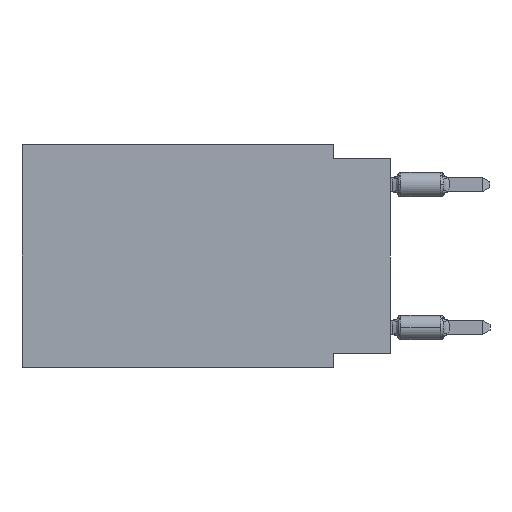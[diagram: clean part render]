
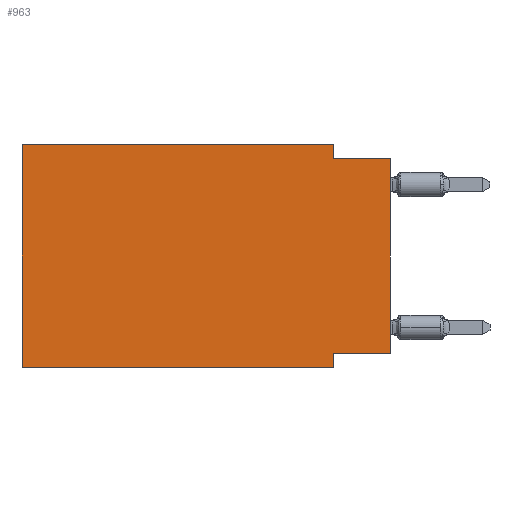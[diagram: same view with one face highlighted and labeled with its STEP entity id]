
A CAD part, left-side view. The second image highlights one B-rep face of the part: STEP entity #963.
In plain terms, the highlighted planar face has unit normal (-1, 0, 0).
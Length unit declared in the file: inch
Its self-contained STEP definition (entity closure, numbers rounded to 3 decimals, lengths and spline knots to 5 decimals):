
#391 = VECTOR ( 'NONE', #8137, 39.37008 ) ;
#597 = VERTEX_POINT ( 'NONE', #22170 ) ;
#775 = CARTESIAN_POINT ( 'NONE',  ( 0., 0.1, -0.39 ) ) ;
#792 = LINE ( 'NONE', #24409, #11663 ) ;
#963 = ADVANCED_FACE ( 'NONE', ( #3192 ), #23662, .F. ) ;
#1130 = DIRECTION ( 'NONE',  ( 0., 0., -1. ) ) ;
#1485 = EDGE_CURVE ( 'NONE', #597, #14681, #17354, .T. ) ;
#1798 = CARTESIAN_POINT ( 'NONE',  ( 0., 0., -0.025 ) ) ;
#2498 = CARTESIAN_POINT ( 'NONE',  ( 0., 0., -0.025 ) ) ;
#2582 = VECTOR ( 'NONE', #13670, 39.37008 ) ;
#2862 = LINE ( 'NONE', #9159, #14213 ) ;
#2925 = ORIENTED_EDGE ( 'NONE', *, *, #15791, .F. ) ;
#3075 = ORIENTED_EDGE ( 'NONE', *, *, #6702, .F. ) ;
#3192 = FACE_OUTER_BOUND ( 'NONE', #8140, .T. ) ;
#4168 = EDGE_CURVE ( 'NONE', #7284, #597, #2862, .T. ) ;
#5283 = LINE ( 'NONE', #15876, #2582 ) ;
#6188 = VECTOR ( 'NONE', #20323, 39.37008 ) ;
#6349 = ORIENTED_EDGE ( 'NONE', *, *, #4168, .F. ) ;
#6597 = CARTESIAN_POINT ( 'NONE',  ( 0., 0.645, -0.39 ) ) ;
#6702 = EDGE_CURVE ( 'NONE', #25868, #7284, #792, .T. ) ;
#7284 = VERTEX_POINT ( 'NONE', #14746 ) ;
#8018 = ORIENTED_EDGE ( 'NONE', *, *, #22584, .T. ) ;
#8137 = DIRECTION ( 'NONE',  ( 0., 1., 0. ) ) ;
#8140 = EDGE_LOOP ( 'NONE', ( #9874, #23512, #26373, #6349, #3075, #8018, #24072, #2925 ) ) ;
#9159 = CARTESIAN_POINT ( 'NONE',  ( 0., 0.645, 0. ) ) ;
#9247 = VERTEX_POINT ( 'NONE', #2498 ) ;
#9703 = DIRECTION ( 'NONE',  ( 0., 0., 1. ) ) ;
#9874 = ORIENTED_EDGE ( 'NONE', *, *, #14035, .T. ) ;
#10467 = CARTESIAN_POINT ( 'NONE',  ( 0., 0., -0.365 ) ) ;
#11663 = VECTOR ( 'NONE', #9703, 39.37008 ) ;
#13018 = VERTEX_POINT ( 'NONE', #22357 ) ;
#13092 = DIRECTION ( 'NONE',  ( 0., 0., -1. ) ) ;
#13108 = EDGE_CURVE ( 'NONE', #15717, #13018, #13531, .T. ) ;
#13531 = LINE ( 'NONE', #775, #24047 ) ;
#13670 = DIRECTION ( 'NONE',  ( 0., 0., 1. ) ) ;
#14035 = EDGE_CURVE ( 'NONE', #26486, #9247, #5283, .T. ) ;
#14213 = VECTOR ( 'NONE', #17275, 39.37008 ) ;
#14681 = VERTEX_POINT ( 'NONE', #20636 ) ;
#14746 = CARTESIAN_POINT ( 'NONE',  ( 0., 0.645, 0. ) ) ;
#15717 = VERTEX_POINT ( 'NONE', #18314 ) ;
#15791 = EDGE_CURVE ( 'NONE', #26486, #15717, #22843, .T. ) ;
#15876 = CARTESIAN_POINT ( 'NONE',  ( 0., 0., 0. ) ) ;
#17275 = DIRECTION ( 'NONE',  ( 0., -1., 0. ) ) ;
#17354 = LINE ( 'NONE', #25895, #23177 ) ;
#17622 = CARTESIAN_POINT ( 'NONE',  ( 0., 0.645, 0. ) ) ;
#18314 = CARTESIAN_POINT ( 'NONE',  ( 0., 0.1, -0.365 ) ) ;
#18888 = DIRECTION ( 'NONE',  ( 0., -1., 0. ) ) ;
#19033 = LINE ( 'NONE', #21077, #26914 ) ;
#20323 = DIRECTION ( 'NONE',  ( 0., -1., 0. ) ) ;
#20636 = CARTESIAN_POINT ( 'NONE',  ( 0., 0.1, -0.025 ) ) ;
#20737 = LINE ( 'NONE', #1798, #6188 ) ;
#21077 = CARTESIAN_POINT ( 'NONE',  ( 0., 0.645, -0.39 ) ) ;
#21614 = EDGE_CURVE ( 'NONE', #14681, #9247, #20737, .T. ) ;
#21926 = DIRECTION ( 'NONE',  ( 0., 0., -1. ) ) ;
#22013 = DIRECTION ( 'NONE',  ( 1., 0., 0. ) ) ;
#22170 = CARTESIAN_POINT ( 'NONE',  ( 0., 0.1, 0. ) ) ;
#22357 = CARTESIAN_POINT ( 'NONE',  ( 0., 0.1, -0.39 ) ) ;
#22584 = EDGE_CURVE ( 'NONE', #25868, #13018, #19033, .T. ) ;
#22762 = AXIS2_PLACEMENT_3D ( 'NONE', #17622, #22013, #1130 ) ;
#22843 = LINE ( 'NONE', #10467, #391 ) ;
#23177 = VECTOR ( 'NONE', #13092, 39.37008 ) ;
#23512 = ORIENTED_EDGE ( 'NONE', *, *, #21614, .F. ) ;
#23662 = PLANE ( 'NONE',  #22762 ) ;
#24047 = VECTOR ( 'NONE', #21926, 39.37008 ) ;
#24072 = ORIENTED_EDGE ( 'NONE', *, *, #13108, .F. ) ;
#24409 = CARTESIAN_POINT ( 'NONE',  ( 0., 0.645, 0. ) ) ;
#25868 = VERTEX_POINT ( 'NONE', #6597 ) ;
#25895 = CARTESIAN_POINT ( 'NONE',  ( 0., 0.1, 0. ) ) ;
#26373 = ORIENTED_EDGE ( 'NONE', *, *, #1485, .F. ) ;
#26486 = VERTEX_POINT ( 'NONE', #27156 ) ;
#26914 = VECTOR ( 'NONE', #18888, 39.37008 ) ;
#27156 = CARTESIAN_POINT ( 'NONE',  ( 0., 0., -0.365 ) ) ;
